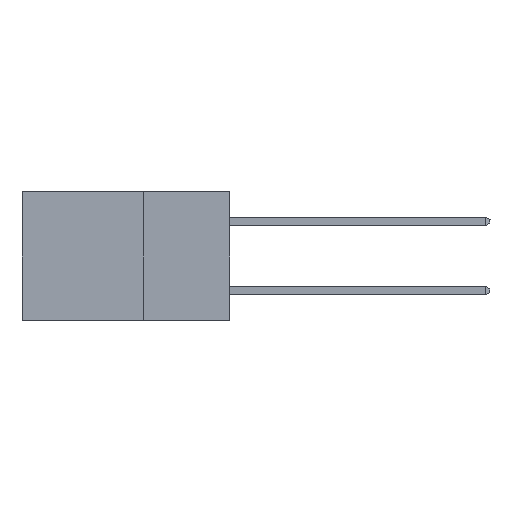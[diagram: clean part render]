
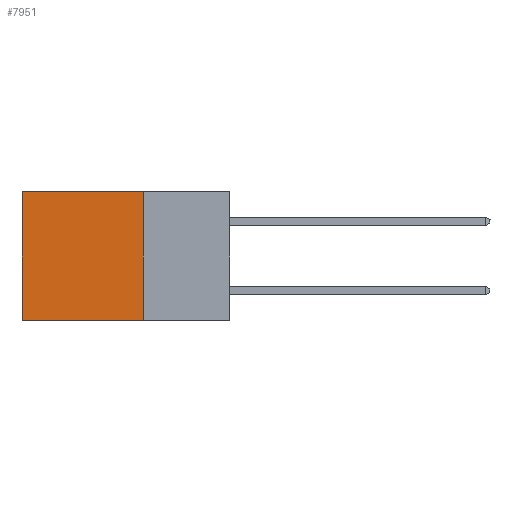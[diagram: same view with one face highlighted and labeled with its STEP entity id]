
A CAD part, left-side view. The second image highlights one B-rep face of the part: STEP entity #7951.
In plain terms, the highlighted planar face has unit normal (-1, 0, 0).
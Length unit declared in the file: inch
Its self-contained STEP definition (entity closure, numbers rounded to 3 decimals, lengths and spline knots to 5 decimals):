
#537 = CARTESIAN_POINT ( 'NONE',  ( 0.2615, 0.25, 0. ) ) ;
#617 = CARTESIAN_POINT ( 'NONE',  ( 0.2615, 0.25, 0. ) ) ;
#726 = DIRECTION ( 'NONE',  ( 0., 1., 0. ) ) ;
#744 = VERTEX_POINT ( 'NONE', #13626 ) ;
#1275 = VERTEX_POINT ( 'NONE', #11130 ) ;
#1671 = LINE ( 'NONE', #8667, #11209 ) ;
#2191 = EDGE_LOOP ( 'NONE', ( #21557, #19586, #21770, #5787 ) ) ;
#3223 = VECTOR ( 'NONE', #726, 39.37008 ) ;
#3368 = EDGE_CURVE ( 'NONE', #5745, #744, #10621, .T. ) ;
#4394 = DIRECTION ( 'NONE',  ( 0., 0., -1. ) ) ;
#5559 = VECTOR ( 'NONE', #8882, 39.37008 ) ;
#5745 = VERTEX_POINT ( 'NONE', #537 ) ;
#5787 = ORIENTED_EDGE ( 'NONE', *, *, #3368, .T. ) ;
#6484 = VERTEX_POINT ( 'NONE', #21814 ) ;
#7717 = FACE_OUTER_BOUND ( 'NONE', #2191, .T. ) ;
#7722 = LINE ( 'NONE', #9495, #9201 ) ;
#7951 = ADVANCED_FACE ( 'NONE', ( #7717 ), #14440, .F. ) ;
#8667 = CARTESIAN_POINT ( 'NONE',  ( 0.2615, 0.25, -0.37 ) ) ;
#8882 = DIRECTION ( 'NONE',  ( 0., 0., -1. ) ) ;
#9201 = VECTOR ( 'NONE', #17912, 39.37008 ) ;
#9228 = EDGE_CURVE ( 'NONE', #6484, #1275, #7722, .T. ) ;
#9495 = CARTESIAN_POINT ( 'NONE',  ( 0.2615, 0.25, -0.37 ) ) ;
#10566 = AXIS2_PLACEMENT_3D ( 'NONE', #21261, #19581, #4394 ) ;
#10621 = LINE ( 'NONE', #617, #3223 ) ;
#11130 = CARTESIAN_POINT ( 'NONE',  ( 0.2615, 0.6, -0.37 ) ) ;
#11209 = VECTOR ( 'NONE', #15167, 39.37008 ) ;
#13626 = CARTESIAN_POINT ( 'NONE',  ( 0.2615, 0.6, 0. ) ) ;
#14440 = PLANE ( 'NONE',  #10566 ) ;
#15167 = DIRECTION ( 'NONE',  ( 0., 0., -1. ) ) ;
#16769 = EDGE_CURVE ( 'NONE', #744, #1275, #17088, .T. ) ;
#16795 = EDGE_CURVE ( 'NONE', #5745, #6484, #1671, .T. ) ;
#17088 = LINE ( 'NONE', #20542, #5559 ) ;
#17912 = DIRECTION ( 'NONE',  ( 0., 1., 0. ) ) ;
#19581 = DIRECTION ( 'NONE',  ( 1., 0., 0. ) ) ;
#19586 = ORIENTED_EDGE ( 'NONE', *, *, #9228, .F. ) ;
#20542 = CARTESIAN_POINT ( 'NONE',  ( 0.2615, 0.6, -0.37 ) ) ;
#21261 = CARTESIAN_POINT ( 'NONE',  ( 0.2615, 0.25, -0.37 ) ) ;
#21557 = ORIENTED_EDGE ( 'NONE', *, *, #16769, .T. ) ;
#21770 = ORIENTED_EDGE ( 'NONE', *, *, #16795, .F. ) ;
#21814 = CARTESIAN_POINT ( 'NONE',  ( 0.2615, 0.25, -0.37 ) ) ;
